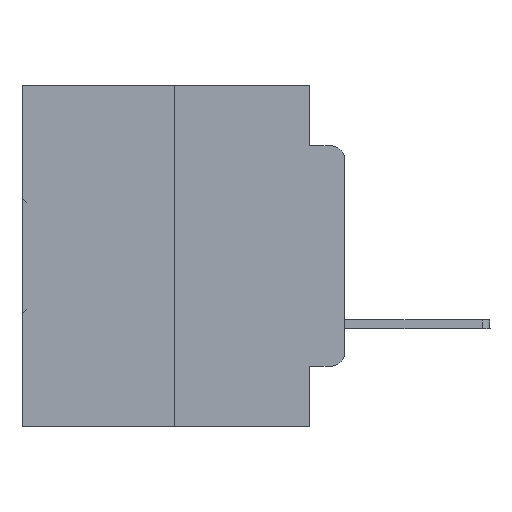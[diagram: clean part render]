
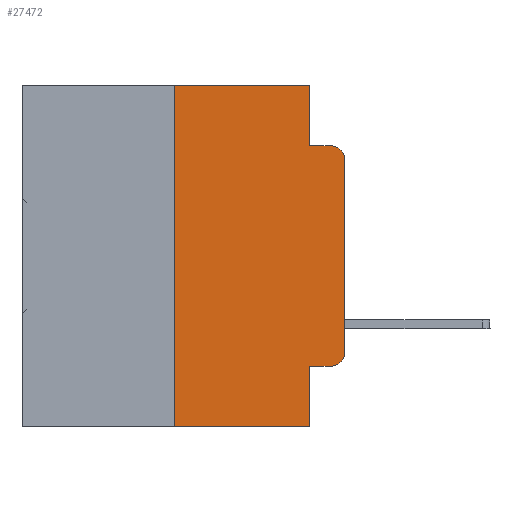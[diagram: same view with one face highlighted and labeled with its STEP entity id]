
A CAD part, left-side view. The second image highlights one B-rep face of the part: STEP entity #27472.
In plain terms, the highlighted planar face has unit normal (-1, 0, 0).
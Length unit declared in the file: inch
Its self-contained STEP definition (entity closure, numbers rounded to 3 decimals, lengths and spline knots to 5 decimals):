
#1299 = CARTESIAN_POINT ( 'NONE',  ( 0., 0.051, -0.4115 ) ) ;
#1351 = VERTEX_POINT ( 'NONE', #27888 ) ;
#1510 = LINE ( 'NONE', #23498, #28148 ) ;
#1946 = EDGE_CURVE ( 'NONE', #22314, #11841, #26703, .T. ) ;
#1996 = LINE ( 'NONE', #1299, #28653 ) ;
#2422 = DIRECTION ( 'NONE',  ( 0., -1., 0. ) ) ;
#2529 = VERTEX_POINT ( 'NONE', #29153 ) ;
#2802 = DIRECTION ( 'NONE',  ( 1., 0., 0. ) ) ;
#3177 = CARTESIAN_POINT ( 'NONE',  ( 0., 0., -0.1085 ) ) ;
#3205 = CARTESIAN_POINT ( 'NONE',  ( 0., 0.02, -0.4115 ) ) ;
#3578 = CARTESIAN_POINT ( 'NONE',  ( 0., 0.02, -0.1085 ) ) ;
#4049 = ORIENTED_EDGE ( 'NONE', *, *, #30352, .T. ) ;
#4225 = VERTEX_POINT ( 'NONE', #3205 ) ;
#4290 = LINE ( 'NONE', #4441, #9430 ) ;
#4441 = CARTESIAN_POINT ( 'NONE',  ( 0., 0.473, 0. ) ) ;
#4513 = EDGE_CURVE ( 'NONE', #11841, #1351, #4290, .T. ) ;
#4674 = FACE_OUTER_BOUND ( 'NONE', #19416, .T. ) ;
#4812 = CARTESIAN_POINT ( 'NONE',  ( 0., 0.25, -0.5 ) ) ;
#5139 = DIRECTION ( 'NONE',  ( 0., 0., -1. ) ) ;
#5317 = CARTESIAN_POINT ( 'NONE',  ( 0., 0.473, -0.5 ) ) ;
#5570 = VECTOR ( 'NONE', #15633, 39.37008 ) ;
#6239 = EDGE_CURVE ( 'NONE', #24099, #25022, #27556, .T. ) ;
#6583 = ORIENTED_EDGE ( 'NONE', *, *, #4513, .F. ) ;
#6856 = DIRECTION ( 'NONE',  ( -1., 0., 0. ) ) ;
#7168 = CIRCLE ( 'NONE', #26615, 0.02 ) ;
#7745 = CIRCLE ( 'NONE', #33054, 0.02 ) ;
#7850 = DIRECTION ( 'NONE',  ( 0., -1., 0. ) ) ;
#7980 = CARTESIAN_POINT ( 'NONE',  ( 0., 0.051, -0.0885 ) ) ;
#8317 = LINE ( 'NONE', #5317, #26678 ) ;
#8473 = DIRECTION ( 'NONE',  ( 0., 0., -1. ) ) ;
#8655 = DIRECTION ( 'NONE',  ( -1., 0., 0. ) ) ;
#8903 = CARTESIAN_POINT ( 'NONE',  ( 0., 0., 0. ) ) ;
#9402 = CARTESIAN_POINT ( 'NONE',  ( 0., 0.051, -0.0885 ) ) ;
#9430 = VECTOR ( 'NONE', #29722, 39.37008 ) ;
#9449 = EDGE_CURVE ( 'NONE', #28506, #2529, #31685, .T. ) ;
#9766 = ORIENTED_EDGE ( 'NONE', *, *, #20494, .T. ) ;
#11021 = DIRECTION ( 'NONE',  ( 0., 0., -1. ) ) ;
#11841 = VERTEX_POINT ( 'NONE', #19598 ) ;
#12023 = CARTESIAN_POINT ( 'NONE',  ( 0., 0.051, -0.5 ) ) ;
#12184 = ORIENTED_EDGE ( 'NONE', *, *, #9449, .F. ) ;
#13004 = LINE ( 'NONE', #20352, #22154 ) ;
#13839 = ORIENTED_EDGE ( 'NONE', *, *, #1946, .F. ) ;
#14192 = DIRECTION ( 'NONE',  ( 0., 0., 1. ) ) ;
#15573 = CARTESIAN_POINT ( 'NONE',  ( 0., 0., -0.3915 ) ) ;
#15633 = DIRECTION ( 'NONE',  ( 0., 0., 1. ) ) ;
#15996 = ORIENTED_EDGE ( 'NONE', *, *, #6239, .T. ) ;
#17201 = ORIENTED_EDGE ( 'NONE', *, *, #25624, .T. ) ;
#18042 = PLANE ( 'NONE',  #18669 ) ;
#18669 = AXIS2_PLACEMENT_3D ( 'NONE', #20689, #2802, #20585 ) ;
#19380 = ORIENTED_EDGE ( 'NONE', *, *, #23665, .T. ) ;
#19416 = EDGE_LOOP ( 'NONE', ( #15996, #4049, #12184, #29150, #6583, #13839, #17201, #28285, #19380, #9766 ) ) ;
#19598 = CARTESIAN_POINT ( 'NONE',  ( 0., 0.25, 0. ) ) ;
#19698 = VERTEX_POINT ( 'NONE', #25705 ) ;
#20352 = CARTESIAN_POINT ( 'NONE',  ( 0., 0.051, 0. ) ) ;
#20494 = EDGE_CURVE ( 'NONE', #4225, #24099, #7745, .T. ) ;
#20585 = DIRECTION ( 'NONE',  ( 0., 0., -1. ) ) ;
#20689 = CARTESIAN_POINT ( 'NONE',  ( 0., 0.473, 0. ) ) ;
#21892 = VERTEX_POINT ( 'NONE', #12023 ) ;
#22154 = VECTOR ( 'NONE', #5139, 39.37008 ) ;
#22314 = VERTEX_POINT ( 'NONE', #4812 ) ;
#22339 = VECTOR ( 'NONE', #14192, 39.37008 ) ;
#22868 = VECTOR ( 'NONE', #2422, 39.37008 ) ;
#23498 = CARTESIAN_POINT ( 'NONE',  ( 0., 0.051, 0. ) ) ;
#23665 = EDGE_CURVE ( 'NONE', #19698, #4225, #1996, .T. ) ;
#24099 = VERTEX_POINT ( 'NONE', #15573 ) ;
#24312 = DIRECTION ( 'NONE',  ( 0., -1., 0. ) ) ;
#25022 = VERTEX_POINT ( 'NONE', #3177 ) ;
#25624 = EDGE_CURVE ( 'NONE', #22314, #21892, #8317, .T. ) ;
#25705 = CARTESIAN_POINT ( 'NONE',  ( 0., 0.051, -0.4115 ) ) ;
#26615 = AXIS2_PLACEMENT_3D ( 'NONE', #3578, #8655, #11021 ) ;
#26678 = VECTOR ( 'NONE', #7850, 39.37008 ) ;
#26703 = LINE ( 'NONE', #32756, #5570 ) ;
#27472 = ADVANCED_FACE ( 'NONE', ( #4674 ), #18042, .F. ) ;
#27556 = LINE ( 'NONE', #8903, #22339 ) ;
#27888 = CARTESIAN_POINT ( 'NONE',  ( 0., 0.051, 0. ) ) ;
#28148 = VECTOR ( 'NONE', #8473, 39.37008 ) ;
#28285 = ORIENTED_EDGE ( 'NONE', *, *, #28405, .F. ) ;
#28405 = EDGE_CURVE ( 'NONE', #19698, #21892, #13004, .T. ) ;
#28506 = VERTEX_POINT ( 'NONE', #7980 ) ;
#28653 = VECTOR ( 'NONE', #24312, 39.37008 ) ;
#29150 = ORIENTED_EDGE ( 'NONE', *, *, #32541, .F. ) ;
#29153 = CARTESIAN_POINT ( 'NONE',  ( 0., 0.02, -0.0885 ) ) ;
#29631 = CARTESIAN_POINT ( 'NONE',  ( 0., 0.02, -0.3915 ) ) ;
#29722 = DIRECTION ( 'NONE',  ( 0., -1., 0. ) ) ;
#30352 = EDGE_CURVE ( 'NONE', #25022, #2529, #7168, .T. ) ;
#31685 = LINE ( 'NONE', #9402, #22868 ) ;
#32404 = DIRECTION ( 'NONE',  ( 0., 0., -1. ) ) ;
#32541 = EDGE_CURVE ( 'NONE', #1351, #28506, #1510, .T. ) ;
#32756 = CARTESIAN_POINT ( 'NONE',  ( 0., 0.25, 0. ) ) ;
#33054 = AXIS2_PLACEMENT_3D ( 'NONE', #29631, #6856, #32404 ) ;
